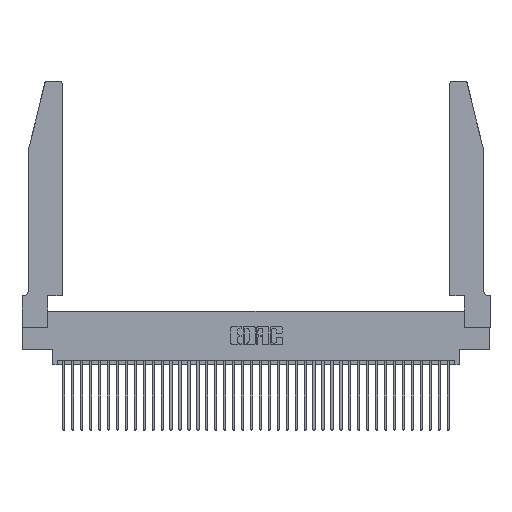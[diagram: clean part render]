
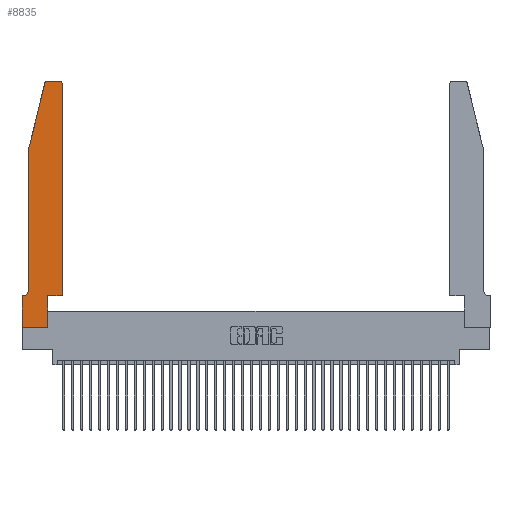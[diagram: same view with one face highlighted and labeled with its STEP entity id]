
A CAD part, top view. The second image highlights one B-rep face of the part: STEP entity #8835.
In plain terms, the highlighted planar face has unit normal (0, 0, 1).
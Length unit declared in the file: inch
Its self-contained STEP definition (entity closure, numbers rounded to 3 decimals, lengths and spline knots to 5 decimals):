
#957 = ORIENTED_EDGE ( 'NONE', *, *, #14722, .T. ) ;
#1508 = VERTEX_POINT ( 'NONE', #24757 ) ;
#2604 = CARTESIAN_POINT ( 'NONE',  ( 0.4505, 0.35, 0.37 ) ) ;
#2731 = CARTESIAN_POINT ( 'NONE',  ( 0.2605, 2.75, 0.37 ) ) ;
#2829 = DIRECTION ( 'NONE',  ( -1., 0., 0. ) ) ;
#3005 = EDGE_CURVE ( 'NONE', #16207, #23305, #14047, .T. ) ;
#3485 = ORIENTED_EDGE ( 'NONE', *, *, #12400, .T. ) ;
#3550 = DIRECTION ( 'NONE',  ( 0., 1., 0. ) ) ;
#4551 = ORIENTED_EDGE ( 'NONE', *, *, #4955, .T. ) ;
#4955 = EDGE_CURVE ( 'NONE', #20736, #16207, #38965, .T. ) ;
#5299 = EDGE_CURVE ( 'NONE', #22079, #35221, #23802, .T. ) ;
#5679 = ORIENTED_EDGE ( 'NONE', *, *, #25410, .T. ) ;
#5748 = CARTESIAN_POINT ( 'NONE',  ( 0.2865, 0.35, 0.37 ) ) ;
#5925 = DIRECTION ( 'NONE',  ( 0., 0., 1. ) ) ;
#6200 = CARTESIAN_POINT ( 'NONE',  ( 0.284, 2.75, 0.37 ) ) ;
#6970 = CARTESIAN_POINT ( 'NONE',  ( 0., 0.35, 0.37 ) ) ;
#6998 = FACE_OUTER_BOUND ( 'NONE', #15778, .T. ) ;
#7453 = ORIENTED_EDGE ( 'NONE', *, *, #3005, .T. ) ;
#7529 = CARTESIAN_POINT ( 'NONE',  ( 0.25487, 2.72718, 0.37 ) ) ;
#8238 = DIRECTION ( 'NONE',  ( 1., 0., 0. ) ) ;
#8835 = ADVANCED_FACE ( 'NONE', ( #6998 ), #12548, .T. ) ;
#8852 = CARTESIAN_POINT ( 'NONE',  ( 0.0755, 0.35, 0.37 ) ) ;
#9419 = DIRECTION ( 'NONE',  ( 0., -1., 0. ) ) ;
#9441 = ORIENTED_EDGE ( 'NONE', *, *, #29552, .T. ) ;
#9535 = CARTESIAN_POINT ( 'NONE',  ( 0.0755, 2., 0.37 ) ) ;
#9928 = CARTESIAN_POINT ( 'NONE',  ( 0., 0.35, 0.37 ) ) ;
#10252 = CARTESIAN_POINT ( 'NONE',  ( 0.0055, 0.35, 0.37 ) ) ;
#10854 = ORIENTED_EDGE ( 'NONE', *, *, #34340, .T. ) ;
#11223 = VECTOR ( 'NONE', #9419, 39.37008 ) ;
#11230 = DIRECTION ( 'NONE',  ( 0., -1., 0. ) ) ;
#12396 = AXIS2_PLACEMENT_3D ( 'NONE', #6970, #21501, #21888 ) ;
#12400 = EDGE_CURVE ( 'NONE', #24786, #1508, #26809, .T. ) ;
#12548 = PLANE ( 'NONE',  #12396 ) ;
#12587 = DIRECTION ( 'NONE',  ( 0., 0., -1. ) ) ;
#13432 = CARTESIAN_POINT ( 'NONE',  ( 0., 0., 0.37 ) ) ;
#13929 = VERTEX_POINT ( 'NONE', #16700 ) ;
#13968 = VERTEX_POINT ( 'NONE', #13432 ) ;
#14047 = LINE ( 'NONE', #29189, #31553 ) ;
#14134 = CARTESIAN_POINT ( 'NONE',  ( 0., 0., 0.37 ) ) ;
#14722 = EDGE_CURVE ( 'NONE', #1508, #21105, #21921, .T. ) ;
#15759 = VERTEX_POINT ( 'NONE', #34428 ) ;
#15778 = EDGE_LOOP ( 'NONE', ( #957, #10854, #4551, #7453, #23321, #25664, #5679, #9441, #35106, #35850, #34616, #3485 ) ) ;
#16207 = VERTEX_POINT ( 'NONE', #9535 ) ;
#16387 = CARTESIAN_POINT ( 'NONE',  ( 0.0755, 0.42, 0.37 ) ) ;
#16700 = CARTESIAN_POINT ( 'NONE',  ( 0.2865, 0., 0.37 ) ) ;
#17390 = DIRECTION ( 'NONE',  ( 0., 1., 0. ) ) ;
#17738 = CARTESIAN_POINT ( 'NONE',  ( 0.284, 2.72, 0.37 ) ) ;
#18063 = DIRECTION ( 'NONE',  ( -1., 0., 0. ) ) ;
#18307 = LINE ( 'NONE', #18527, #11223 ) ;
#18527 = CARTESIAN_POINT ( 'NONE',  ( 0., 0., 0.37 ) ) ;
#18715 = CARTESIAN_POINT ( 'NONE',  ( 0.4505, 0.35, 0.37 ) ) ;
#19417 = CARTESIAN_POINT ( 'NONE',  ( 0.0055, 0.42, 0.37 ) ) ;
#19950 = VERTEX_POINT ( 'NONE', #18715 ) ;
#20585 = VECTOR ( 'NONE', #17390, 39.37008 ) ;
#20626 = CARTESIAN_POINT ( 'NONE',  ( 0.4505, 2.72, 0.37 ) ) ;
#20736 = VERTEX_POINT ( 'NONE', #7529 ) ;
#20909 = DIRECTION ( 'NONE',  ( 0., 0., 1. ) ) ;
#21005 = DIRECTION ( 'NONE',  ( 1., 0., 0. ) ) ;
#21105 = VERTEX_POINT ( 'NONE', #6200 ) ;
#21138 = VECTOR ( 'NONE', #3550, 39.37008 ) ;
#21174 = LINE ( 'NONE', #14134, #23516 ) ;
#21183 = EDGE_CURVE ( 'NONE', #19950, #24786, #24430, .T. ) ;
#21501 = DIRECTION ( 'NONE',  ( 0., 0., 1. ) ) ;
#21661 = CIRCLE ( 'NONE', #23763, 0.07 ) ;
#21888 = DIRECTION ( 'NONE',  ( 1., 0., 0. ) ) ;
#21921 = LINE ( 'NONE', #2731, #25244 ) ;
#22079 = VERTEX_POINT ( 'NONE', #10252 ) ;
#22967 = DIRECTION ( 'NONE',  ( 1., 0., 0. ) ) ;
#23305 = VERTEX_POINT ( 'NONE', #16387 ) ;
#23321 = ORIENTED_EDGE ( 'NONE', *, *, #33949, .T. ) ;
#23388 = CARTESIAN_POINT ( 'NONE',  ( 0.0755, 2., 0.37 ) ) ;
#23516 = VECTOR ( 'NONE', #22967, 39.37008 ) ;
#23763 = AXIS2_PLACEMENT_3D ( 'NONE', #19417, #12587, #25518 ) ;
#23802 = LINE ( 'NONE', #8852, #34730 ) ;
#23888 = LINE ( 'NONE', #5748, #20585 ) ;
#24430 = LINE ( 'NONE', #30787, #21138 ) ;
#24757 = CARTESIAN_POINT ( 'NONE',  ( 0.4205, 2.75, 0.37 ) ) ;
#24786 = VERTEX_POINT ( 'NONE', #20626 ) ;
#25244 = VECTOR ( 'NONE', #18063, 39.37008 ) ;
#25410 = EDGE_CURVE ( 'NONE', #35221, #13968, #18307, .T. ) ;
#25518 = DIRECTION ( 'NONE',  ( -1., 0., 0. ) ) ;
#25664 = ORIENTED_EDGE ( 'NONE', *, *, #5299, .T. ) ;
#26331 = EDGE_CURVE ( 'NONE', #13929, #15759, #23888, .T. ) ;
#26809 = CIRCLE ( 'NONE', #37751, 0.03 ) ;
#27019 = VECTOR ( 'NONE', #32509, 39.37008 ) ;
#29189 = CARTESIAN_POINT ( 'NONE',  ( 0.0755, 2., 0.37 ) ) ;
#29552 = EDGE_CURVE ( 'NONE', #13968, #13929, #21174, .T. ) ;
#30787 = CARTESIAN_POINT ( 'NONE',  ( 0.4505, 0.35, 0.37 ) ) ;
#31553 = VECTOR ( 'NONE', #11230, 39.37008 ) ;
#32132 = DIRECTION ( 'NONE',  ( -0.239, -0.971, 0. ) ) ;
#32509 = DIRECTION ( 'NONE',  ( 1., 0., 0. ) ) ;
#33949 = EDGE_CURVE ( 'NONE', #23305, #22079, #21661, .T. ) ;
#34340 = EDGE_CURVE ( 'NONE', #21105, #20736, #34438, .T. ) ;
#34428 = CARTESIAN_POINT ( 'NONE',  ( 0.2865, 0.35, 0.37 ) ) ;
#34438 = CIRCLE ( 'NONE', #36477, 0.03 ) ;
#34616 = ORIENTED_EDGE ( 'NONE', *, *, #21183, .T. ) ;
#34730 = VECTOR ( 'NONE', #2829, 39.37008 ) ;
#35106 = ORIENTED_EDGE ( 'NONE', *, *, #26331, .T. ) ;
#35221 = VERTEX_POINT ( 'NONE', #9928 ) ;
#35529 = LINE ( 'NONE', #2604, #27019 ) ;
#35850 = ORIENTED_EDGE ( 'NONE', *, *, #38137, .T. ) ;
#36096 = CARTESIAN_POINT ( 'NONE',  ( 0.4205, 2.72, 0.37 ) ) ;
#36477 = AXIS2_PLACEMENT_3D ( 'NONE', #17738, #20909, #8238 ) ;
#36570 = VECTOR ( 'NONE', #32132, 39.37008 ) ;
#37751 = AXIS2_PLACEMENT_3D ( 'NONE', #36096, #5925, #21005 ) ;
#38137 = EDGE_CURVE ( 'NONE', #15759, #19950, #35529, .T. ) ;
#38965 = LINE ( 'NONE', #23388, #36570 ) ;
